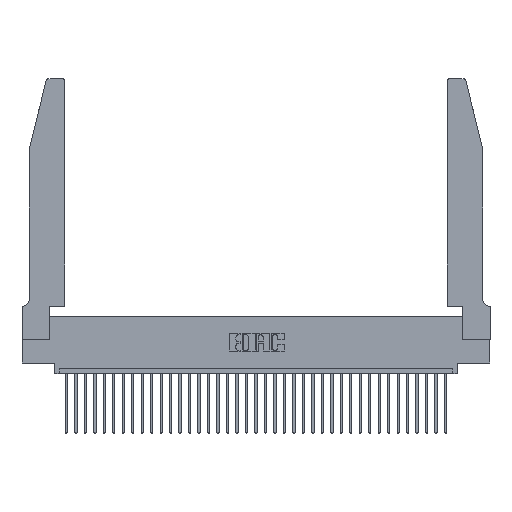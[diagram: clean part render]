
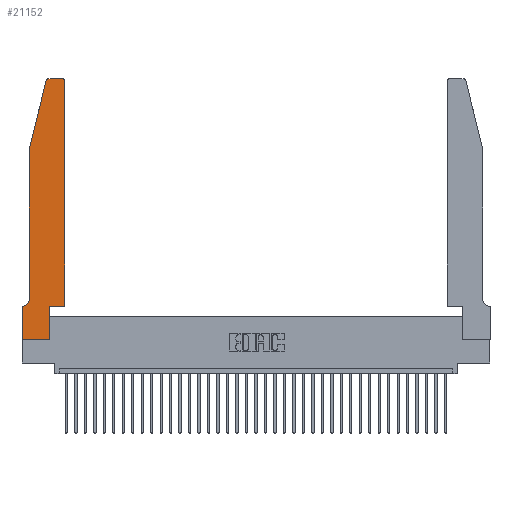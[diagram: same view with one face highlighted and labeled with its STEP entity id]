
A CAD part, top view. The second image highlights one B-rep face of the part: STEP entity #21152.
In plain terms, the highlighted planar face has unit normal (0, 0, 1).
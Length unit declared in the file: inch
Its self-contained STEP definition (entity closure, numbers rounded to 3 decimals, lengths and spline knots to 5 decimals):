
#92 = PLANE ( 'NONE',  #2878 ) ;
#2307 = CARTESIAN_POINT ( 'NONE',  ( 0.284, 2.75, 0.37 ) ) ;
#2878 = AXIS2_PLACEMENT_3D ( 'NONE', #19539, #22513, #3008 ) ;
#3008 = DIRECTION ( 'NONE',  ( 1., 0., 0. ) ) ;
#3354 = DIRECTION ( 'NONE',  ( -1., 0., 0. ) ) ;
#3788 = LINE ( 'NONE', #7551, #35017 ) ;
#3854 = CARTESIAN_POINT ( 'NONE',  ( 0.4205, 2.72, 0.37 ) ) ;
#4812 = EDGE_CURVE ( 'NONE', #32132, #6041, #30196, .T. ) ;
#5126 = VERTEX_POINT ( 'NONE', #11353 ) ;
#5695 = VERTEX_POINT ( 'NONE', #18963 ) ;
#6041 = VERTEX_POINT ( 'NONE', #32054 ) ;
#6325 = CARTESIAN_POINT ( 'NONE',  ( 0.4505, 0.35, 0.37 ) ) ;
#6408 = AXIS2_PLACEMENT_3D ( 'NONE', #29785, #18297, #34971 ) ;
#6979 = VERTEX_POINT ( 'NONE', #29839 ) ;
#7551 = CARTESIAN_POINT ( 'NONE',  ( 0., 0., 0.37 ) ) ;
#7802 = VECTOR ( 'NONE', #29019, 39.37008 ) ;
#7891 = ORIENTED_EDGE ( 'NONE', *, *, #23899, .T. ) ;
#8361 = DIRECTION ( 'NONE',  ( 1., 0., 0. ) ) ;
#8891 = DIRECTION ( 'NONE',  ( 1., 0., 0. ) ) ;
#9368 = VERTEX_POINT ( 'NONE', #31498 ) ;
#10067 = DIRECTION ( 'NONE',  ( 1., 0., 0. ) ) ;
#10094 = DIRECTION ( 'NONE',  ( 0., -1., 0. ) ) ;
#10365 = CARTESIAN_POINT ( 'NONE',  ( 0.25487, 2.72718, 0.37 ) ) ;
#10818 = EDGE_CURVE ( 'NONE', #5126, #23349, #11308, .T. ) ;
#10979 = CARTESIAN_POINT ( 'NONE',  ( 0.0755, 2., 0.37 ) ) ;
#11308 = LINE ( 'NONE', #18800, #13104 ) ;
#11353 = CARTESIAN_POINT ( 'NONE',  ( 0.2865, 0., 0.37 ) ) ;
#11756 = CARTESIAN_POINT ( 'NONE',  ( 0.4505, 2.72, 0.37 ) ) ;
#11981 = VECTOR ( 'NONE', #15047, 39.37008 ) ;
#12826 = VECTOR ( 'NONE', #24629, 39.37008 ) ;
#12903 = CARTESIAN_POINT ( 'NONE',  ( 0.2605, 2.75, 0.37 ) ) ;
#13104 = VECTOR ( 'NONE', #33027, 39.37008 ) ;
#13356 = CARTESIAN_POINT ( 'NONE',  ( 0.0755, 2., 0.37 ) ) ;
#13792 = EDGE_CURVE ( 'NONE', #20576, #32705, #15198, .T. ) ;
#13864 = EDGE_CURVE ( 'NONE', #32705, #34079, #30302, .T. ) ;
#14849 = EDGE_CURVE ( 'NONE', #5695, #32132, #25868, .T. ) ;
#14923 = CARTESIAN_POINT ( 'NONE',  ( 0., 0., 0.37 ) ) ;
#15047 = DIRECTION ( 'NONE',  ( 1., 0., 0. ) ) ;
#15089 = LINE ( 'NONE', #6325, #15525 ) ;
#15198 = LINE ( 'NONE', #25974, #7802 ) ;
#15525 = VECTOR ( 'NONE', #8891, 39.37008 ) ;
#15572 = EDGE_LOOP ( 'NONE', ( #24758, #20214, #35233, #7891, #22816, #28444, #20536, #23414, #16883, #30786, #22236, #18768 ) ) ;
#16883 = ORIENTED_EDGE ( 'NONE', *, *, #10818, .T. ) ;
#18132 = VECTOR ( 'NONE', #27318, 39.37008 ) ;
#18297 = DIRECTION ( 'NONE',  ( 0., 0., -1. ) ) ;
#18768 = ORIENTED_EDGE ( 'NONE', *, *, #13864, .T. ) ;
#18800 = CARTESIAN_POINT ( 'NONE',  ( 0.2865, 0.35, 0.37 ) ) ;
#18861 = EDGE_CURVE ( 'NONE', #19361, #9368, #24473, .T. ) ;
#18963 = CARTESIAN_POINT ( 'NONE',  ( 0.0755, 0.42, 0.37 ) ) ;
#19003 = LINE ( 'NONE', #13356, #18132 ) ;
#19361 = VERTEX_POINT ( 'NONE', #10365 ) ;
#19539 = CARTESIAN_POINT ( 'NONE',  ( 0., 0.35, 0.37 ) ) ;
#20214 = ORIENTED_EDGE ( 'NONE', *, *, #33678, .T. ) ;
#20535 = CIRCLE ( 'NONE', #24455, 0.03 ) ;
#20536 = ORIENTED_EDGE ( 'NONE', *, *, #22813, .T. ) ;
#20576 = VERTEX_POINT ( 'NONE', #22666 ) ;
#20816 = AXIS2_PLACEMENT_3D ( 'NONE', #3854, #32083, #10067 ) ;
#21152 = ADVANCED_FACE ( 'NONE', ( #26121 ), #92, .T. ) ;
#21200 = CARTESIAN_POINT ( 'NONE',  ( 0.4205, 2.75, 0.37 ) ) ;
#21344 = DIRECTION ( 'NONE',  ( -1., 0., 0. ) ) ;
#22236 = ORIENTED_EDGE ( 'NONE', *, *, #13792, .T. ) ;
#22269 = CARTESIAN_POINT ( 'NONE',  ( 0.2865, 0.35, 0.37 ) ) ;
#22513 = DIRECTION ( 'NONE',  ( 0., 0., 1. ) ) ;
#22666 = CARTESIAN_POINT ( 'NONE',  ( 0.4505, 0.35, 0.37 ) ) ;
#22813 = EDGE_CURVE ( 'NONE', #6041, #6979, #3788, .T. ) ;
#22816 = ORIENTED_EDGE ( 'NONE', *, *, #14849, .T. ) ;
#23297 = VERTEX_POINT ( 'NONE', #2307 ) ;
#23349 = VERTEX_POINT ( 'NONE', #22269 ) ;
#23414 = ORIENTED_EDGE ( 'NONE', *, *, #31455, .T. ) ;
#23899 = EDGE_CURVE ( 'NONE', #9368, #5695, #19003, .T. ) ;
#24175 = EDGE_CURVE ( 'NONE', #23349, #20576, #15089, .T. ) ;
#24455 = AXIS2_PLACEMENT_3D ( 'NONE', #24944, #27825, #8361 ) ;
#24473 = LINE ( 'NONE', #10979, #12826 ) ;
#24629 = DIRECTION ( 'NONE',  ( -0.239, -0.971, 0. ) ) ;
#24758 = ORIENTED_EDGE ( 'NONE', *, *, #25527, .T. ) ;
#24944 = CARTESIAN_POINT ( 'NONE',  ( 0.284, 2.72, 0.37 ) ) ;
#25527 = EDGE_CURVE ( 'NONE', #34079, #23297, #30123, .T. ) ;
#25868 = CIRCLE ( 'NONE', #6408, 0.07 ) ;
#25974 = CARTESIAN_POINT ( 'NONE',  ( 0.4505, 0.35, 0.37 ) ) ;
#26121 = FACE_OUTER_BOUND ( 'NONE', #15572, .T. ) ;
#27318 = DIRECTION ( 'NONE',  ( 0., -1., 0. ) ) ;
#27562 = VECTOR ( 'NONE', #3354, 39.37008 ) ;
#27825 = DIRECTION ( 'NONE',  ( 0., 0., 1. ) ) ;
#28444 = ORIENTED_EDGE ( 'NONE', *, *, #4812, .T. ) ;
#29019 = DIRECTION ( 'NONE',  ( 0., 1., 0. ) ) ;
#29785 = CARTESIAN_POINT ( 'NONE',  ( 0.0055, 0.42, 0.37 ) ) ;
#29839 = CARTESIAN_POINT ( 'NONE',  ( 0., 0., 0.37 ) ) ;
#30123 = LINE ( 'NONE', #12903, #32720 ) ;
#30196 = LINE ( 'NONE', #32390, #27562 ) ;
#30302 = CIRCLE ( 'NONE', #20816, 0.03 ) ;
#30786 = ORIENTED_EDGE ( 'NONE', *, *, #24175, .T. ) ;
#31455 = EDGE_CURVE ( 'NONE', #6979, #5126, #32794, .T. ) ;
#31498 = CARTESIAN_POINT ( 'NONE',  ( 0.0755, 2., 0.37 ) ) ;
#32054 = CARTESIAN_POINT ( 'NONE',  ( 0., 0.35, 0.37 ) ) ;
#32083 = DIRECTION ( 'NONE',  ( 0., 0., 1. ) ) ;
#32132 = VERTEX_POINT ( 'NONE', #34469 ) ;
#32390 = CARTESIAN_POINT ( 'NONE',  ( 0.0755, 0.35, 0.37 ) ) ;
#32705 = VERTEX_POINT ( 'NONE', #11756 ) ;
#32720 = VECTOR ( 'NONE', #21344, 39.37008 ) ;
#32794 = LINE ( 'NONE', #14923, #11981 ) ;
#33027 = DIRECTION ( 'NONE',  ( 0., 1., 0. ) ) ;
#33678 = EDGE_CURVE ( 'NONE', #23297, #19361, #20535, .T. ) ;
#34079 = VERTEX_POINT ( 'NONE', #21200 ) ;
#34469 = CARTESIAN_POINT ( 'NONE',  ( 0.0055, 0.35, 0.37 ) ) ;
#34971 = DIRECTION ( 'NONE',  ( -1., 0., 0. ) ) ;
#35017 = VECTOR ( 'NONE', #10094, 39.37008 ) ;
#35233 = ORIENTED_EDGE ( 'NONE', *, *, #18861, .T. ) ;
